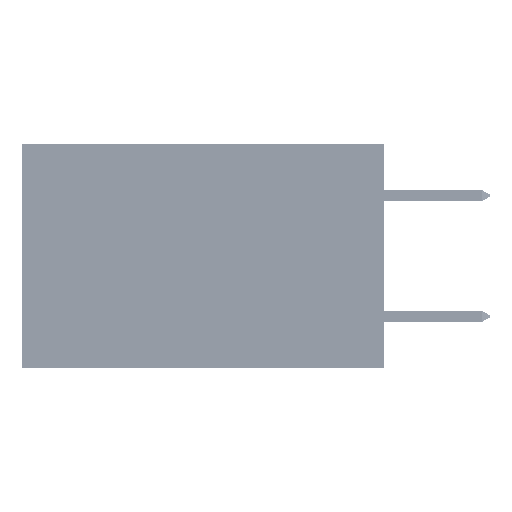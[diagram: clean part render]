
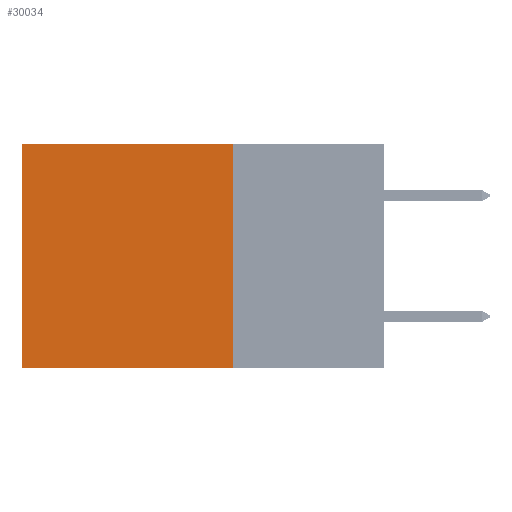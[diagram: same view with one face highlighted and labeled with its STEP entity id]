
A CAD part, left-side view. The second image highlights one B-rep face of the part: STEP entity #30034.
In plain terms, the highlighted planar face has unit normal (-1, 0, 0).
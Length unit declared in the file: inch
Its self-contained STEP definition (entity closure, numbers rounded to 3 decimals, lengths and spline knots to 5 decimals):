
#12 = LINE ( 'NONE', #33543, #38801 ) ;
#864 = EDGE_CURVE ( 'NONE', #20108, #13726, #2048, .T. ) ;
#1938 = DIRECTION ( 'NONE',  ( 1., 0., 0. ) ) ;
#2048 = LINE ( 'NONE', #11994, #21436 ) ;
#2353 = VERTEX_POINT ( 'NONE', #16318 ) ;
#3094 = DIRECTION ( 'NONE',  ( 0., 1., 0. ) ) ;
#3661 = AXIS2_PLACEMENT_3D ( 'NONE', #32208, #1938, #43738 ) ;
#8813 = LINE ( 'NONE', #29422, #25915 ) ;
#9763 = CARTESIAN_POINT ( 'NONE',  ( 0.2875, 0.25, 0. ) ) ;
#10719 = EDGE_LOOP ( 'NONE', ( #27589, #46639, #14799, #17685 ) ) ;
#11994 = CARTESIAN_POINT ( 'NONE',  ( 0.2875, 0.25, 0. ) ) ;
#13726 = VERTEX_POINT ( 'NONE', #34406 ) ;
#14137 = EDGE_CURVE ( 'NONE', #13726, #2353, #8813, .T. ) ;
#14799 = ORIENTED_EDGE ( 'NONE', *, *, #33000, .F. ) ;
#16318 = CARTESIAN_POINT ( 'NONE',  ( 0.2875, 0.6, -0.37 ) ) ;
#17685 = ORIENTED_EDGE ( 'NONE', *, *, #864, .T. ) ;
#18390 = EDGE_CURVE ( 'NONE', #23949, #2353, #12, .T. ) ;
#18481 = DIRECTION ( 'NONE',  ( 0., 1., 0. ) ) ;
#20108 = VERTEX_POINT ( 'NONE', #45720 ) ;
#20770 = LINE ( 'NONE', #9763, #22508 ) ;
#21436 = VECTOR ( 'NONE', #18481, 39.37008 ) ;
#22508 = VECTOR ( 'NONE', #36104, 39.37008 ) ;
#23949 = VERTEX_POINT ( 'NONE', #25585 ) ;
#25585 = CARTESIAN_POINT ( 'NONE',  ( 0.2875, 0.25, -0.37 ) ) ;
#25915 = VECTOR ( 'NONE', #44104, 39.37008 ) ;
#27589 = ORIENTED_EDGE ( 'NONE', *, *, #14137, .T. ) ;
#29422 = CARTESIAN_POINT ( 'NONE',  ( 0.2875, 0.6, 0. ) ) ;
#30034 = ADVANCED_FACE ( 'NONE', ( #32037 ), #36170, .F. ) ;
#32037 = FACE_OUTER_BOUND ( 'NONE', #10719, .T. ) ;
#32208 = CARTESIAN_POINT ( 'NONE',  ( 0.2875, 0.25, 0. ) ) ;
#33000 = EDGE_CURVE ( 'NONE', #20108, #23949, #20770, .T. ) ;
#33543 = CARTESIAN_POINT ( 'NONE',  ( 0.2875, 0.25, -0.37 ) ) ;
#34406 = CARTESIAN_POINT ( 'NONE',  ( 0.2875, 0.6, 0. ) ) ;
#36104 = DIRECTION ( 'NONE',  ( 0., 0., -1. ) ) ;
#36170 = PLANE ( 'NONE',  #3661 ) ;
#38801 = VECTOR ( 'NONE', #3094, 39.37008 ) ;
#43738 = DIRECTION ( 'NONE',  ( 0., 0., -1. ) ) ;
#44104 = DIRECTION ( 'NONE',  ( 0., 0., -1. ) ) ;
#45720 = CARTESIAN_POINT ( 'NONE',  ( 0.2875, 0.25, 0. ) ) ;
#46639 = ORIENTED_EDGE ( 'NONE', *, *, #18390, .F. ) ;
